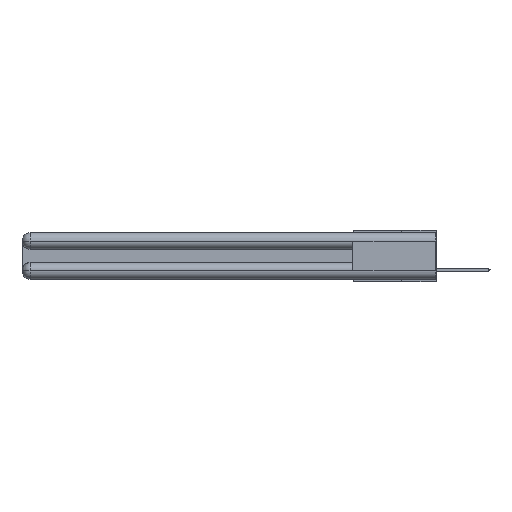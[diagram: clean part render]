
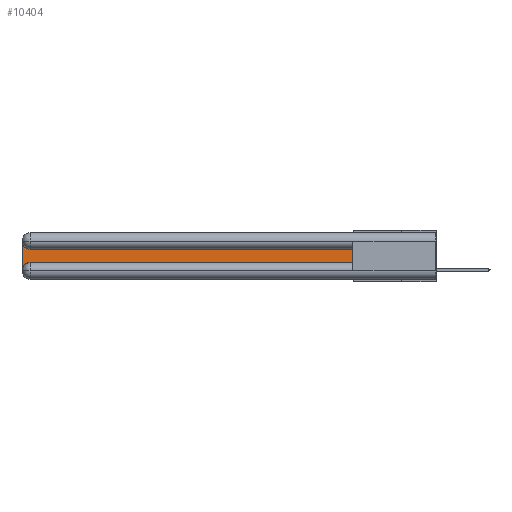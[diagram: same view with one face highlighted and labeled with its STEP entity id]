
A CAD part, left-side view. The second image highlights one B-rep face of the part: STEP entity #10404.
In plain terms, the highlighted planar face has unit normal (-1, 0, 0).
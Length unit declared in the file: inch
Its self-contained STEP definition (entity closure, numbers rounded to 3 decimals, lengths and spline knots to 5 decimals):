
#433 = CARTESIAN_POINT ( 'NONE',  ( 0.075, 0.6, -0.2175 ) ) ;
#1419 = AXIS2_PLACEMENT_3D ( 'NONE', #30869, #14910, #22728 ) ;
#1515 = EDGE_CURVE ( 'NONE', #1969, #5206, #30024, .T. ) ;
#1964 = EDGE_CURVE ( 'NONE', #12608, #14102, #19554, .T. ) ;
#1969 = VERTEX_POINT ( 'NONE', #27857 ) ;
#3260 = ORIENTED_EDGE ( 'NONE', *, *, #32884, .T. ) ;
#4245 = VECTOR ( 'NONE', #19370, 39.37008 ) ;
#4531 = VECTOR ( 'NONE', #24740, 39.37008 ) ;
#5206 = VERTEX_POINT ( 'NONE', #29963 ) ;
#5504 = CARTESIAN_POINT ( 'NONE',  ( 0.075, 2.94, -0.0625 ) ) ;
#6122 = CARTESIAN_POINT ( 'NONE',  ( 0.075, 0.6, -0.2175 ) ) ;
#6397 = EDGE_CURVE ( 'NONE', #14102, #19001, #33749, .T. ) ;
#7134 = CIRCLE ( 'NONE', #22240, 0.06 ) ;
#7567 = ORIENTED_EDGE ( 'NONE', *, *, #6397, .T. ) ;
#9011 = CARTESIAN_POINT ( 'NONE',  ( 0.075, 3., -0.2175 ) ) ;
#9193 = PLANE ( 'NONE',  #33592 ) ;
#10404 = ADVANCED_FACE ( 'NONE', ( #24699 ), #9193, .F. ) ;
#11219 = CARTESIAN_POINT ( 'NONE',  ( 0.075, 0.6, -0.2175 ) ) ;
#11884 = DIRECTION ( 'NONE',  ( 1., 0., 0. ) ) ;
#12608 = VERTEX_POINT ( 'NONE', #21302 ) ;
#13473 = DIRECTION ( 'NONE',  ( 0., 0., 1. ) ) ;
#13900 = DIRECTION ( 'NONE',  ( 0., 0., -1. ) ) ;
#14102 = VERTEX_POINT ( 'NONE', #30630 ) ;
#14415 = ORIENTED_EDGE ( 'NONE', *, *, #17987, .T. ) ;
#14619 = DIRECTION ( 'NONE',  ( 0., 1., 0. ) ) ;
#14910 = DIRECTION ( 'NONE',  ( 1., 0., 0. ) ) ;
#16113 = ORIENTED_EDGE ( 'NONE', *, *, #1964, .T. ) ;
#17565 = LINE ( 'NONE', #6122, #4245 ) ;
#17653 = ORIENTED_EDGE ( 'NONE', *, *, #1515, .T. ) ;
#17987 = EDGE_CURVE ( 'NONE', #29603, #1969, #30642, .T. ) ;
#19001 = VERTEX_POINT ( 'NONE', #19697 ) ;
#19370 = DIRECTION ( 'NONE',  ( 0., -1., 0. ) ) ;
#19554 = LINE ( 'NONE', #9011, #4531 ) ;
#19697 = CARTESIAN_POINT ( 'NONE',  ( 0.075, 2.94, -0.2175 ) ) ;
#21302 = CARTESIAN_POINT ( 'NONE',  ( 0.075, 3., -0.0625 ) ) ;
#22240 = AXIS2_PLACEMENT_3D ( 'NONE', #5504, #24262, #13900 ) ;
#22728 = DIRECTION ( 'NONE',  ( 0., 0., -1. ) ) ;
#22773 = CARTESIAN_POINT ( 'NONE',  ( 0.075, 0.6, -0.1225 ) ) ;
#22909 = VECTOR ( 'NONE', #14619, 39.37008 ) ;
#23567 = VECTOR ( 'NONE', #13473, 39.37008 ) ;
#24262 = DIRECTION ( 'NONE',  ( 1., 0., 0. ) ) ;
#24699 = FACE_OUTER_BOUND ( 'NONE', #25007, .T. ) ;
#24740 = DIRECTION ( 'NONE',  ( 0., 0., -1. ) ) ;
#25007 = EDGE_LOOP ( 'NONE', ( #17653, #3260, #16113, #7567, #29217, #14415 ) ) ;
#27857 = CARTESIAN_POINT ( 'NONE',  ( 0.075, 0.6, -0.1225 ) ) ;
#29217 = ORIENTED_EDGE ( 'NONE', *, *, #32231, .T. ) ;
#29603 = VERTEX_POINT ( 'NONE', #11219 ) ;
#29963 = CARTESIAN_POINT ( 'NONE',  ( 0.075, 2.94, -0.1225 ) ) ;
#30024 = LINE ( 'NONE', #22773, #22909 ) ;
#30630 = CARTESIAN_POINT ( 'NONE',  ( 0.075, 3., -0.2775 ) ) ;
#30642 = LINE ( 'NONE', #433, #23567 ) ;
#30738 = CARTESIAN_POINT ( 'NONE',  ( 0.075, 3., -0.1225 ) ) ;
#30869 = CARTESIAN_POINT ( 'NONE',  ( 0.075, 2.94, -0.2775 ) ) ;
#32231 = EDGE_CURVE ( 'NONE', #19001, #29603, #17565, .T. ) ;
#32884 = EDGE_CURVE ( 'NONE', #5206, #12608, #7134, .T. ) ;
#33295 = DIRECTION ( 'NONE',  ( 0., 0., -1. ) ) ;
#33592 = AXIS2_PLACEMENT_3D ( 'NONE', #30738, #11884, #33295 ) ;
#33749 = CIRCLE ( 'NONE', #1419, 0.06 ) ;
